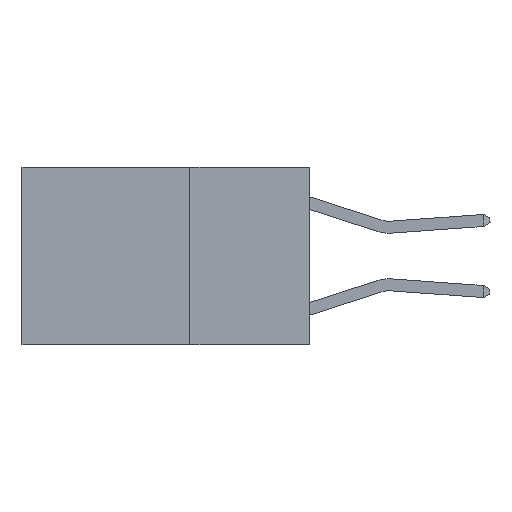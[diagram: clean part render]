
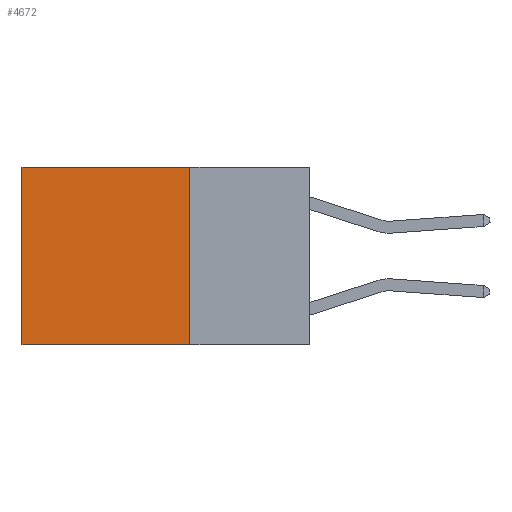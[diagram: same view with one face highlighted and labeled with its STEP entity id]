
A CAD part, left-side view. The second image highlights one B-rep face of the part: STEP entity #4672.
In plain terms, the highlighted planar face has unit normal (-1, 0, 0).
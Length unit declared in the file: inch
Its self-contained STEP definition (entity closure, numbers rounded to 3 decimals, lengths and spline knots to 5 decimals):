
#198 = CARTESIAN_POINT ( 'NONE',  ( 0.2625, 0.25, 0. ) ) ;
#206 = CARTESIAN_POINT ( 'NONE',  ( 0.2625, 0.25, 0. ) ) ;
#439 = DIRECTION ( 'NONE',  ( 0., 1., 0. ) ) ;
#620 = LINE ( 'NONE', #10673, #10273 ) ;
#1182 = DIRECTION ( 'NONE',  ( 0., 0., -1. ) ) ;
#1353 = LINE ( 'NONE', #2498, #3943 ) ;
#1934 = EDGE_CURVE ( 'NONE', #9362, #11288, #620, .T. ) ;
#2498 = CARTESIAN_POINT ( 'NONE',  ( 0.2625, 0.25, 0. ) ) ;
#3148 = DIRECTION ( 'NONE',  ( 0., 0., -1. ) ) ;
#3512 = DIRECTION ( 'NONE',  ( 0., 1., 0. ) ) ;
#3534 = CARTESIAN_POINT ( 'NONE',  ( 0.2625, 0.6, 0. ) ) ;
#3868 = VECTOR ( 'NONE', #3148, 39.37008 ) ;
#3943 = VECTOR ( 'NONE', #3512, 39.37008 ) ;
#4383 = FACE_OUTER_BOUND ( 'NONE', #4445, .T. ) ;
#4445 = EDGE_LOOP ( 'NONE', ( #5739, #8127, #6031, #10706 ) ) ;
#4672 = ADVANCED_FACE ( 'NONE', ( #4383 ), #11332, .F. ) ;
#4980 = CARTESIAN_POINT ( 'NONE',  ( 0.2625, 0.25, -0.37 ) ) ;
#5088 = AXIS2_PLACEMENT_3D ( 'NONE', #198, #6973, #1182 ) ;
#5491 = VERTEX_POINT ( 'NONE', #3534 ) ;
#5739 = ORIENTED_EDGE ( 'NONE', *, *, #10013, .T. ) ;
#6031 = ORIENTED_EDGE ( 'NONE', *, *, #11615, .F. ) ;
#6715 = LINE ( 'NONE', #206, #10831 ) ;
#6973 = DIRECTION ( 'NONE',  ( 1., 0., 0. ) ) ;
#7879 = DIRECTION ( 'NONE',  ( 0., 0., -1. ) ) ;
#8127 = ORIENTED_EDGE ( 'NONE', *, *, #1934, .F. ) ;
#8344 = CARTESIAN_POINT ( 'NONE',  ( 0.2625, 0.6, -0.37 ) ) ;
#8849 = LINE ( 'NONE', #11406, #3868 ) ;
#9013 = EDGE_CURVE ( 'NONE', #10436, #5491, #1353, .T. ) ;
#9243 = CARTESIAN_POINT ( 'NONE',  ( 0.2625, 0.25, 0. ) ) ;
#9362 = VERTEX_POINT ( 'NONE', #4980 ) ;
#10013 = EDGE_CURVE ( 'NONE', #5491, #11288, #8849, .T. ) ;
#10273 = VECTOR ( 'NONE', #439, 39.37008 ) ;
#10436 = VERTEX_POINT ( 'NONE', #9243 ) ;
#10673 = CARTESIAN_POINT ( 'NONE',  ( 0.2625, 0.25, -0.37 ) ) ;
#10706 = ORIENTED_EDGE ( 'NONE', *, *, #9013, .T. ) ;
#10831 = VECTOR ( 'NONE', #7879, 39.37008 ) ;
#11288 = VERTEX_POINT ( 'NONE', #8344 ) ;
#11332 = PLANE ( 'NONE',  #5088 ) ;
#11406 = CARTESIAN_POINT ( 'NONE',  ( 0.2625, 0.6, 0. ) ) ;
#11615 = EDGE_CURVE ( 'NONE', #10436, #9362, #6715, .T. ) ;
